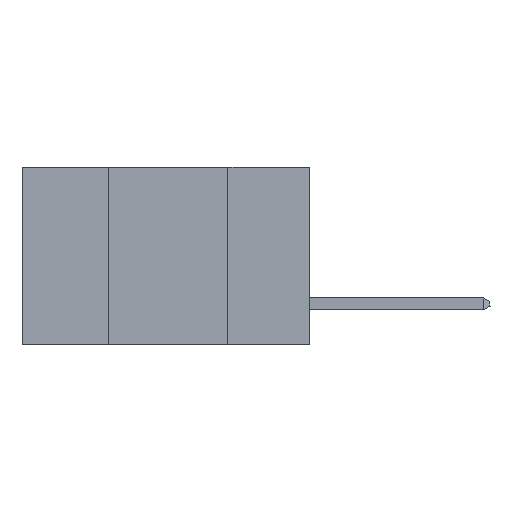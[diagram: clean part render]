
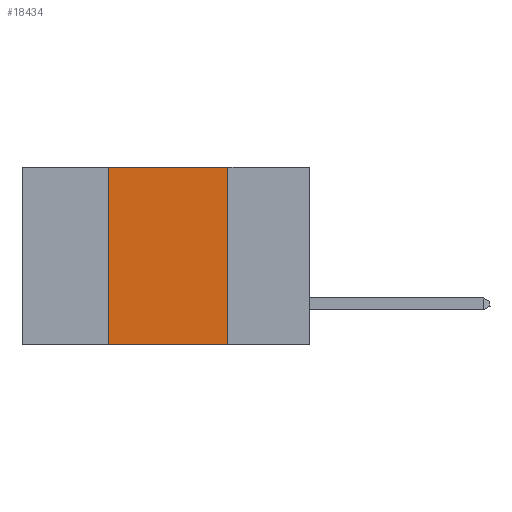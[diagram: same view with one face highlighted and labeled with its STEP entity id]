
A CAD part, left-side view. The second image highlights one B-rep face of the part: STEP entity #18434.
In plain terms, the highlighted planar face has unit normal (-1, 0, 0).
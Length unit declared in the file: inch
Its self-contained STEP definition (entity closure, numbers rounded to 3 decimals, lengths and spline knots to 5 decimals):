
#423 = CARTESIAN_POINT ( 'NONE',  ( 0., 0.6, -0.37 ) ) ;
#2387 = CARTESIAN_POINT ( 'NONE',  ( 0., 0.6, 0. ) ) ;
#3927 = ORIENTED_EDGE ( 'NONE', *, *, #29646, .F. ) ;
#5416 = VERTEX_POINT ( 'NONE', #24288 ) ;
#6572 = LINE ( 'NONE', #423, #14339 ) ;
#6857 = EDGE_CURVE ( 'NONE', #33706, #23155, #14766, .T. ) ;
#7399 = DIRECTION ( 'NONE',  ( 0., -1., 0. ) ) ;
#7712 = FACE_OUTER_BOUND ( 'NONE', #7751, .T. ) ;
#7751 = EDGE_LOOP ( 'NONE', ( #3927, #19631, #28319, #35594 ) ) ;
#10417 = LINE ( 'NONE', #21271, #13523 ) ;
#13523 = VECTOR ( 'NONE', #31390, 39.37008 ) ;
#14339 = VECTOR ( 'NONE', #36857, 39.37008 ) ;
#14600 = CARTESIAN_POINT ( 'NONE',  ( 0., 0.42, 0. ) ) ;
#14766 = LINE ( 'NONE', #34263, #18402 ) ;
#18402 = VECTOR ( 'NONE', #7399, 39.37008 ) ;
#18434 = ADVANCED_FACE ( 'NONE', ( #7712 ), #38416, .F. ) ;
#19631 = ORIENTED_EDGE ( 'NONE', *, *, #6857, .F. ) ;
#21271 = CARTESIAN_POINT ( 'NONE',  ( 0., 0.17, 0. ) ) ;
#23087 = VERTEX_POINT ( 'NONE', #35896 ) ;
#23155 = VERTEX_POINT ( 'NONE', #38307 ) ;
#23999 = CARTESIAN_POINT ( 'NONE',  ( 0., 0.42, 0. ) ) ;
#24179 = EDGE_CURVE ( 'NONE', #23087, #33706, #29690, .T. ) ;
#24288 = CARTESIAN_POINT ( 'NONE',  ( 0., 0.17, -0.37 ) ) ;
#25597 = DIRECTION ( 'NONE',  ( 0., 0., -1. ) ) ;
#26483 = EDGE_CURVE ( 'NONE', #23087, #5416, #6572, .T. ) ;
#28319 = ORIENTED_EDGE ( 'NONE', *, *, #24179, .F. ) ;
#29286 = AXIS2_PLACEMENT_3D ( 'NONE', #2387, #38689, #25597 ) ;
#29646 = EDGE_CURVE ( 'NONE', #23155, #5416, #10417, .T. ) ;
#29690 = LINE ( 'NONE', #14600, #33761 ) ;
#31390 = DIRECTION ( 'NONE',  ( 0., 0., -1. ) ) ;
#33706 = VERTEX_POINT ( 'NONE', #23999 ) ;
#33761 = VECTOR ( 'NONE', #40258, 39.37008 ) ;
#34263 = CARTESIAN_POINT ( 'NONE',  ( 0., 0.6, 0. ) ) ;
#35594 = ORIENTED_EDGE ( 'NONE', *, *, #26483, .T. ) ;
#35896 = CARTESIAN_POINT ( 'NONE',  ( 0., 0.42, -0.37 ) ) ;
#36857 = DIRECTION ( 'NONE',  ( 0., -1., 0. ) ) ;
#38307 = CARTESIAN_POINT ( 'NONE',  ( 0., 0.17, 0. ) ) ;
#38416 = PLANE ( 'NONE',  #29286 ) ;
#38689 = DIRECTION ( 'NONE',  ( 1., 0., 0. ) ) ;
#40258 = DIRECTION ( 'NONE',  ( 0., 0., 1. ) ) ;
